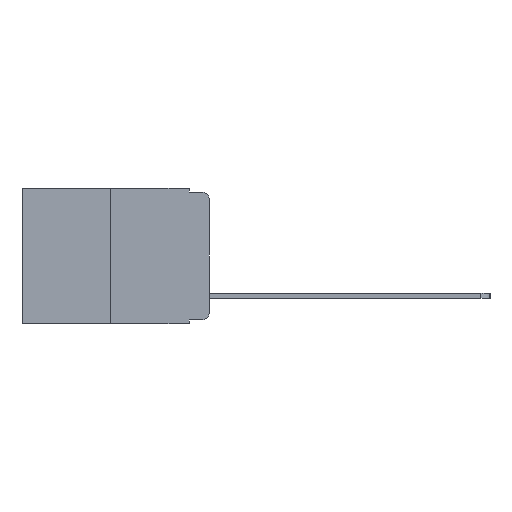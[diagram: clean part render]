
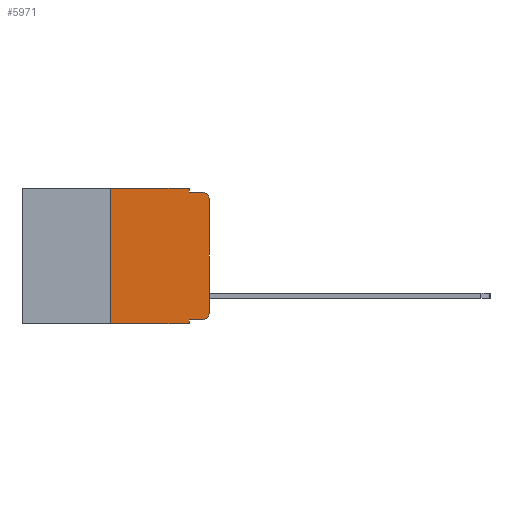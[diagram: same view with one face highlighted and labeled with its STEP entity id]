
A CAD part, left-side view. The second image highlights one B-rep face of the part: STEP entity #5971.
In plain terms, the highlighted planar face has unit normal (-1, 0, 0).
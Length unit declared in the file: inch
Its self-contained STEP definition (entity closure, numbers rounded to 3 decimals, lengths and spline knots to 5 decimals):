
#396 = EDGE_CURVE ( 'NONE', #3499, #6399, #12202, .T. ) ;
#467 = CARTESIAN_POINT ( 'NONE',  ( 0., 0.051, -0.343 ) ) ;
#515 = CARTESIAN_POINT ( 'NONE',  ( 0., 0.473, -0.343 ) ) ;
#534 = VERTEX_POINT ( 'NONE', #12844 ) ;
#592 = ORIENTED_EDGE ( 'NONE', *, *, #12507, .T. ) ;
#822 = VECTOR ( 'NONE', #11816, 39.37008 ) ;
#1021 = CARTESIAN_POINT ( 'NONE',  ( 0., 0.02, -0.313 ) ) ;
#1183 = ORIENTED_EDGE ( 'NONE', *, *, #18339, .F. ) ;
#1325 = VECTOR ( 'NONE', #19113, 39.37008 ) ;
#1694 = EDGE_CURVE ( 'NONE', #10342, #4641, #7076, .T. ) ;
#1839 = AXIS2_PLACEMENT_3D ( 'NONE', #1021, #14105, #2977 ) ;
#2282 = VERTEX_POINT ( 'NONE', #16627 ) ;
#2437 = ORIENTED_EDGE ( 'NONE', *, *, #20633, .F. ) ;
#2646 = VECTOR ( 'NONE', #18778, 39.37008 ) ;
#2659 = CARTESIAN_POINT ( 'NONE',  ( 0., 0.473, 0. ) ) ;
#2926 = VECTOR ( 'NONE', #4237, 39.37008 ) ;
#2968 = VERTEX_POINT ( 'NONE', #14567 ) ;
#2977 = DIRECTION ( 'NONE',  ( 0., 0., -1. ) ) ;
#3499 = VERTEX_POINT ( 'NONE', #23247 ) ;
#3666 = CARTESIAN_POINT ( 'NONE',  ( 0., 0.473, 0. ) ) ;
#4217 = CIRCLE ( 'NONE', #1839, 0.02 ) ;
#4237 = DIRECTION ( 'NONE',  ( 0., -1., 0. ) ) ;
#4641 = VERTEX_POINT ( 'NONE', #467 ) ;
#4937 = CARTESIAN_POINT ( 'NONE',  ( 0., 0.051, 0. ) ) ;
#5119 = CARTESIAN_POINT ( 'NONE',  ( 0., 0.25, 0. ) ) ;
#5476 = PLANE ( 'NONE',  #9040 ) ;
#5531 = EDGE_CURVE ( 'NONE', #10342, #2968, #7077, .T. ) ;
#5560 = DIRECTION ( 'NONE',  ( 0., 0., -1. ) ) ;
#5612 = CARTESIAN_POINT ( 'NONE',  ( 0., 0., 0. ) ) ;
#5971 = ADVANCED_FACE ( 'NONE', ( #10218 ), #5476, .F. ) ;
#6395 = LINE ( 'NONE', #22682, #1325 ) ;
#6399 = VERTEX_POINT ( 'NONE', #5119 ) ;
#7076 = LINE ( 'NONE', #19480, #822 ) ;
#7077 = LINE ( 'NONE', #17933, #2646 ) ;
#7161 = CARTESIAN_POINT ( 'NONE',  ( 0., 0.051, -0.01 ) ) ;
#7181 = DIRECTION ( 'NONE',  ( -1., 0., 0. ) ) ;
#7509 = DIRECTION ( 'NONE',  ( 0., 0., 1. ) ) ;
#7954 = LINE ( 'NONE', #15347, #2926 ) ;
#8455 = CARTESIAN_POINT ( 'NONE',  ( 0., 0.02, -0.01 ) ) ;
#8893 = ORIENTED_EDGE ( 'NONE', *, *, #16035, .T. ) ;
#9040 = AXIS2_PLACEMENT_3D ( 'NONE', #3666, #16630, #5560 ) ;
#9498 = VECTOR ( 'NONE', #7509, 39.37008 ) ;
#9996 = DIRECTION ( 'NONE',  ( 0., -1., 0. ) ) ;
#10052 = LINE ( 'NONE', #5612, #9498 ) ;
#10218 = FACE_OUTER_BOUND ( 'NONE', #19917, .T. ) ;
#10342 = VERTEX_POINT ( 'NONE', #15497 ) ;
#10503 = EDGE_CURVE ( 'NONE', #2968, #534, #4217, .T. ) ;
#11816 = DIRECTION ( 'NONE',  ( 0., 0., -1. ) ) ;
#12202 = LINE ( 'NONE', #21684, #14354 ) ;
#12332 = ORIENTED_EDGE ( 'NONE', *, *, #1694, .F. ) ;
#12365 = CIRCLE ( 'NONE', #23863, 0.02 ) ;
#12507 = EDGE_CURVE ( 'NONE', #3499, #4641, #14907, .T. ) ;
#12844 = CARTESIAN_POINT ( 'NONE',  ( 0., 0., -0.313 ) ) ;
#13767 = ORIENTED_EDGE ( 'NONE', *, *, #10503, .T. ) ;
#14105 = DIRECTION ( 'NONE',  ( -1., 0., 0. ) ) ;
#14325 = VECTOR ( 'NONE', #9996, 39.37008 ) ;
#14354 = VECTOR ( 'NONE', #19025, 39.37008 ) ;
#14567 = CARTESIAN_POINT ( 'NONE',  ( 0., 0.02, -0.333 ) ) ;
#14601 = VERTEX_POINT ( 'NONE', #7161 ) ;
#14907 = LINE ( 'NONE', #515, #14325 ) ;
#15347 = CARTESIAN_POINT ( 'NONE',  ( 0., 0.051, -0.01 ) ) ;
#15497 = CARTESIAN_POINT ( 'NONE',  ( 0., 0.051, -0.333 ) ) ;
#15528 = ORIENTED_EDGE ( 'NONE', *, *, #15890, .T. ) ;
#15890 = EDGE_CURVE ( 'NONE', #2282, #16991, #12365, .T. ) ;
#16035 = EDGE_CURVE ( 'NONE', #534, #2282, #10052, .T. ) ;
#16089 = ORIENTED_EDGE ( 'NONE', *, *, #396, .F. ) ;
#16627 = CARTESIAN_POINT ( 'NONE',  ( 0., 0., -0.03 ) ) ;
#16630 = DIRECTION ( 'NONE',  ( 1., 0., 0. ) ) ;
#16991 = VERTEX_POINT ( 'NONE', #8455 ) ;
#17933 = CARTESIAN_POINT ( 'NONE',  ( 0., 0.051, -0.333 ) ) ;
#18180 = CARTESIAN_POINT ( 'NONE',  ( 0., 0.02, -0.03 ) ) ;
#18339 = EDGE_CURVE ( 'NONE', #14601, #16991, #7954, .T. ) ;
#18778 = DIRECTION ( 'NONE',  ( 0., -1., 0. ) ) ;
#19000 = VECTOR ( 'NONE', #21044, 39.37008 ) ;
#19025 = DIRECTION ( 'NONE',  ( 0., 0., 1. ) ) ;
#19113 = DIRECTION ( 'NONE',  ( 0., 0., -1. ) ) ;
#19480 = CARTESIAN_POINT ( 'NONE',  ( 0., 0.051, 0. ) ) ;
#19555 = EDGE_CURVE ( 'NONE', #23289, #14601, #6395, .T. ) ;
#19578 = LINE ( 'NONE', #2659, #19000 ) ;
#19917 = EDGE_LOOP ( 'NONE', ( #8893, #15528, #1183, #22323, #2437, #16089, #592, #12332, #22088, #13767 ) ) ;
#20011 = DIRECTION ( 'NONE',  ( 0., 0., -1. ) ) ;
#20633 = EDGE_CURVE ( 'NONE', #6399, #23289, #19578, .T. ) ;
#21044 = DIRECTION ( 'NONE',  ( 0., -1., 0. ) ) ;
#21684 = CARTESIAN_POINT ( 'NONE',  ( 0., 0.25, 0. ) ) ;
#22088 = ORIENTED_EDGE ( 'NONE', *, *, #5531, .T. ) ;
#22323 = ORIENTED_EDGE ( 'NONE', *, *, #19555, .F. ) ;
#22682 = CARTESIAN_POINT ( 'NONE',  ( 0., 0.051, 0. ) ) ;
#23247 = CARTESIAN_POINT ( 'NONE',  ( 0., 0.25, -0.343 ) ) ;
#23289 = VERTEX_POINT ( 'NONE', #4937 ) ;
#23863 = AXIS2_PLACEMENT_3D ( 'NONE', #18180, #7181, #20011 ) ;
